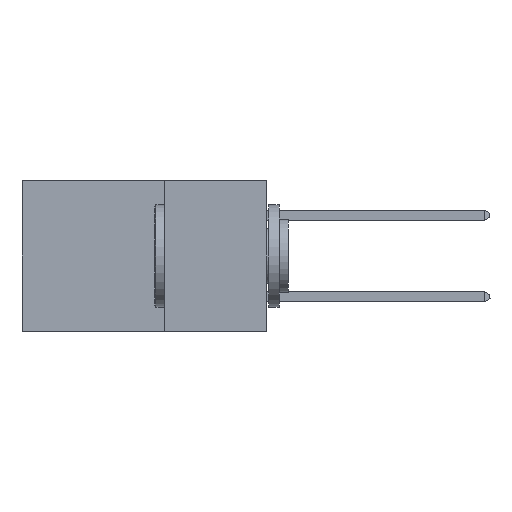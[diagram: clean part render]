
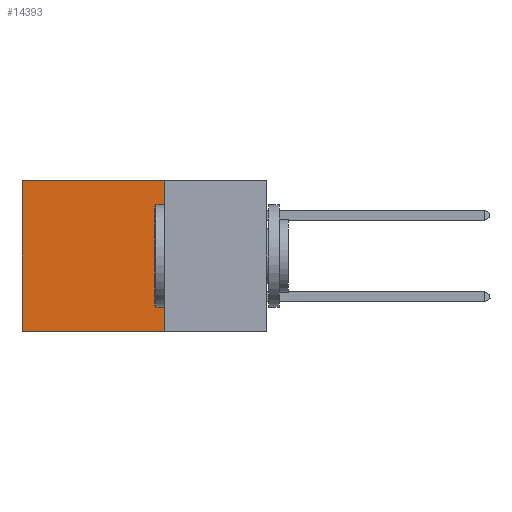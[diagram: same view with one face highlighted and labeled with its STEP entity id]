
A CAD part, left-side view. The second image highlights one B-rep face of the part: STEP entity #14393.
In plain terms, the highlighted planar face has unit normal (-1, 0, 0).
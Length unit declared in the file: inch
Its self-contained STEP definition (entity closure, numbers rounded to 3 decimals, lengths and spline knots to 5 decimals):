
#471 = DIRECTION ( 'NONE',  ( 1., 0., 0. ) ) ;
#897 = CARTESIAN_POINT ( 'NONE',  ( 0.2875, 0.25, 0. ) ) ;
#1441 = FACE_OUTER_BOUND ( 'NONE', #24571, .T. ) ;
#2134 = DIRECTION ( 'NONE',  ( 0., 1., 0. ) ) ;
#3186 = EDGE_CURVE ( 'NONE', #20305, #13484, #24213, .T. ) ;
#4558 = LINE ( 'NONE', #16264, #7028 ) ;
#5226 = EDGE_CURVE ( 'NONE', #6168, #10672, #20083, .T. ) ;
#6168 = VERTEX_POINT ( 'NONE', #897 ) ;
#6656 = LINE ( 'NONE', #23674, #8803 ) ;
#7028 = VECTOR ( 'NONE', #24844, 39.37008 ) ;
#8803 = VECTOR ( 'NONE', #2134, 39.37008 ) ;
#9399 = EDGE_CURVE ( 'NONE', #10672, #13484, #6656, .T. ) ;
#9999 = ORIENTED_EDGE ( 'NONE', *, *, #9399, .F. ) ;
#10096 = CARTESIAN_POINT ( 'NONE',  ( 0.2875, 0.25, 0. ) ) ;
#10418 = ORIENTED_EDGE ( 'NONE', *, *, #19857, .T. ) ;
#10672 = VERTEX_POINT ( 'NONE', #17072 ) ;
#10693 = CARTESIAN_POINT ( 'NONE',  ( 0.2875, 0.6, 0. ) ) ;
#10774 = CARTESIAN_POINT ( 'NONE',  ( 0.2875, 0.25, 0. ) ) ;
#12332 = DIRECTION ( 'NONE',  ( 0., 0., -1. ) ) ;
#13484 = VERTEX_POINT ( 'NONE', #23427 ) ;
#14393 = ADVANCED_FACE ( 'NONE', ( #1441 ), #18692, .F. ) ;
#15184 = ORIENTED_EDGE ( 'NONE', *, *, #5226, .F. ) ;
#15874 = DIRECTION ( 'NONE',  ( 0., 0., -1. ) ) ;
#16264 = CARTESIAN_POINT ( 'NONE',  ( 0.2875, 0.25, 0. ) ) ;
#17072 = CARTESIAN_POINT ( 'NONE',  ( 0.2875, 0.25, -0.37 ) ) ;
#18244 = ORIENTED_EDGE ( 'NONE', *, *, #3186, .T. ) ;
#18299 = VECTOR ( 'NONE', #24778, 39.37008 ) ;
#18692 = PLANE ( 'NONE',  #25456 ) ;
#19471 = VECTOR ( 'NONE', #15874, 39.37008 ) ;
#19857 = EDGE_CURVE ( 'NONE', #6168, #20305, #4558, .T. ) ;
#20083 = LINE ( 'NONE', #10096, #19471 ) ;
#20305 = VERTEX_POINT ( 'NONE', #25803 ) ;
#23427 = CARTESIAN_POINT ( 'NONE',  ( 0.2875, 0.6, -0.37 ) ) ;
#23674 = CARTESIAN_POINT ( 'NONE',  ( 0.2875, 0.25, -0.37 ) ) ;
#24213 = LINE ( 'NONE', #10693, #18299 ) ;
#24571 = EDGE_LOOP ( 'NONE', ( #18244, #9999, #15184, #10418 ) ) ;
#24778 = DIRECTION ( 'NONE',  ( 0., 0., -1. ) ) ;
#24844 = DIRECTION ( 'NONE',  ( 0., 1., 0. ) ) ;
#25456 = AXIS2_PLACEMENT_3D ( 'NONE', #10774, #471, #12332 ) ;
#25803 = CARTESIAN_POINT ( 'NONE',  ( 0.2875, 0.6, 0. ) ) ;
